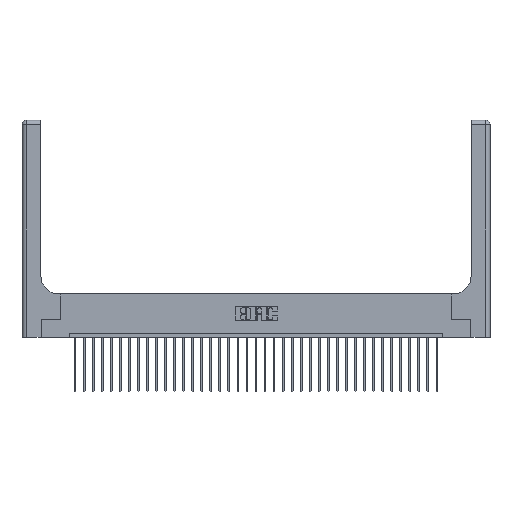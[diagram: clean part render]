
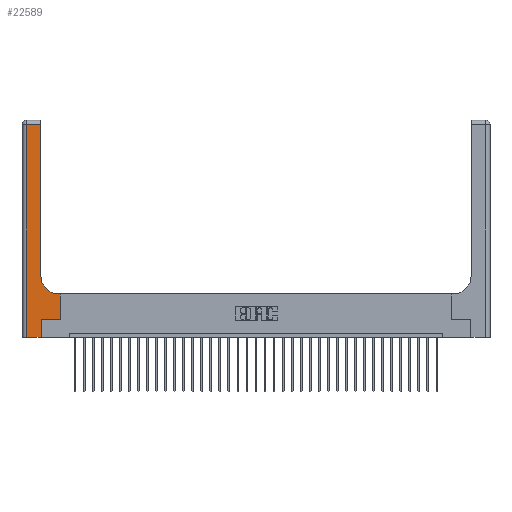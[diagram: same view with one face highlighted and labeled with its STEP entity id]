
A CAD part, top view. The second image highlights one B-rep face of the part: STEP entity #22589.
In plain terms, the highlighted planar face has unit normal (0, 0, 1).
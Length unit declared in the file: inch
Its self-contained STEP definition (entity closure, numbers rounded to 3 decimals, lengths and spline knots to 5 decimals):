
#271 = EDGE_CURVE ( 'NONE', #10063, #20399, #29861, .T. ) ;
#325 = DIRECTION ( 'NONE',  ( 0., 0., -1. ) ) ;
#635 = CARTESIAN_POINT ( 'NONE',  ( 0.06, 2.94, 0.37 ) ) ;
#3884 = EDGE_CURVE ( 'NONE', #7198, #19068, #24522, .T. ) ;
#4706 = VERTEX_POINT ( 'NONE', #23035 ) ;
#4895 = DIRECTION ( 'NONE',  ( -1., 0., 0. ) ) ;
#5053 = VECTOR ( 'NONE', #22862, 39.37008 ) ;
#5226 = CARTESIAN_POINT ( 'NONE',  ( 0.26, 2.94, 0.37 ) ) ;
#5548 = ORIENTED_EDGE ( 'NONE', *, *, #19573, .T. ) ;
#5899 = LINE ( 'NONE', #7981, #23345 ) ;
#5954 = LINE ( 'NONE', #9879, #23741 ) ;
#6757 = VECTOR ( 'NONE', #23575, 39.37008 ) ;
#7185 = PLANE ( 'NONE',  #28968 ) ;
#7198 = VERTEX_POINT ( 'NONE', #10456 ) ;
#7258 = CARTESIAN_POINT ( 'NONE',  ( 0., 2.94, 0.37 ) ) ;
#7278 = ORIENTED_EDGE ( 'NONE', *, *, #19802, .T. ) ;
#7500 = ORIENTED_EDGE ( 'NONE', *, *, #27510, .T. ) ;
#7981 = CARTESIAN_POINT ( 'NONE',  ( 0.26, 3., 0.37 ) ) ;
#8164 = DIRECTION ( 'NONE',  ( 0., 1., 0. ) ) ;
#8450 = DIRECTION ( 'NONE',  ( 1., 0., 0. ) ) ;
#8610 = VERTEX_POINT ( 'NONE', #23771 ) ;
#8743 = CARTESIAN_POINT ( 'NONE',  ( 0., 0., 0.37 ) ) ;
#9048 = CARTESIAN_POINT ( 'NONE',  ( 0.26, 0.85, 0.37 ) ) ;
#9879 = CARTESIAN_POINT ( 'NONE',  ( 0.26, 0.6, 0.37 ) ) ;
#10063 = VERTEX_POINT ( 'NONE', #18207 ) ;
#10200 = LINE ( 'NONE', #12173, #28010 ) ;
#10275 = CARTESIAN_POINT ( 'NONE',  ( 0.265, 0., 0.37 ) ) ;
#10456 = CARTESIAN_POINT ( 'NONE',  ( 0.265, 0.25, 0.37 ) ) ;
#12022 = CARTESIAN_POINT ( 'NONE',  ( 0.528, 0.25, 0.37 ) ) ;
#12166 = EDGE_LOOP ( 'NONE', ( #25432, #7500, #29569, #5548, #7278, #21839, #30677, #12741, #23522 ) ) ;
#12173 = CARTESIAN_POINT ( 'NONE',  ( 0.06, 3., 0.37 ) ) ;
#12741 = ORIENTED_EDGE ( 'NONE', *, *, #16975, .T. ) ;
#13682 = DIRECTION ( 'NONE',  ( 0., 0., -1. ) ) ;
#14010 = LINE ( 'NONE', #8743, #5053 ) ;
#15401 = CARTESIAN_POINT ( 'NONE',  ( 0.265, 0., 0.37 ) ) ;
#15419 = CARTESIAN_POINT ( 'NONE',  ( 0.528, 0.25, 0.37 ) ) ;
#16135 = VERTEX_POINT ( 'NONE', #5226 ) ;
#16975 = EDGE_CURVE ( 'NONE', #4706, #10063, #5954, .T. ) ;
#17598 = EDGE_CURVE ( 'NONE', #20399, #16135, #5899, .T. ) ;
#17746 = EDGE_CURVE ( 'NONE', #19068, #4706, #30760, .T. ) ;
#18207 = CARTESIAN_POINT ( 'NONE',  ( 0.51, 0.6, 0.37 ) ) ;
#19068 = VERTEX_POINT ( 'NONE', #12022 ) ;
#19573 = EDGE_CURVE ( 'NONE', #8610, #22750, #14010, .T. ) ;
#19642 = DIRECTION ( 'NONE',  ( -1., 0., 0. ) ) ;
#19802 = EDGE_CURVE ( 'NONE', #22750, #7198, #26176, .T. ) ;
#19907 = VECTOR ( 'NONE', #8164, 39.37008 ) ;
#20399 = VERTEX_POINT ( 'NONE', #9048 ) ;
#20532 = EDGE_CURVE ( 'NONE', #26271, #8610, #10200, .T. ) ;
#20753 = VECTOR ( 'NONE', #25188, 39.37008 ) ;
#21287 = DIRECTION ( 'NONE',  ( -1., 0., 0. ) ) ;
#21786 = DIRECTION ( 'NONE',  ( 0., -1., 0. ) ) ;
#21839 = ORIENTED_EDGE ( 'NONE', *, *, #3884, .T. ) ;
#22589 = ADVANCED_FACE ( 'NONE', ( #29532 ), #7185, .F. ) ;
#22750 = VERTEX_POINT ( 'NONE', #15401 ) ;
#22862 = DIRECTION ( 'NONE',  ( 1., 0., 0. ) ) ;
#22871 = CARTESIAN_POINT ( 'NONE',  ( 0.51, 0.85, 0.37 ) ) ;
#23035 = CARTESIAN_POINT ( 'NONE',  ( 0.528, 0.6, 0.37 ) ) ;
#23345 = VECTOR ( 'NONE', #26850, 39.37008 ) ;
#23522 = ORIENTED_EDGE ( 'NONE', *, *, #271, .T. ) ;
#23575 = DIRECTION ( 'NONE',  ( 1., 0., 0. ) ) ;
#23741 = VECTOR ( 'NONE', #19642, 39.37008 ) ;
#23771 = CARTESIAN_POINT ( 'NONE',  ( 0.06, 0., 0.37 ) ) ;
#23787 = CARTESIAN_POINT ( 'NONE',  ( 0., 3., 0.37 ) ) ;
#24386 = VECTOR ( 'NONE', #21287, 39.37008 ) ;
#24522 = LINE ( 'NONE', #28549, #6757 ) ;
#25188 = DIRECTION ( 'NONE',  ( 0., 1., 0. ) ) ;
#25432 = ORIENTED_EDGE ( 'NONE', *, *, #17598, .T. ) ;
#26176 = LINE ( 'NONE', #10275, #19907 ) ;
#26271 = VERTEX_POINT ( 'NONE', #635 ) ;
#26850 = DIRECTION ( 'NONE',  ( 0., 1., 0. ) ) ;
#27510 = EDGE_CURVE ( 'NONE', #16135, #26271, #30753, .T. ) ;
#28010 = VECTOR ( 'NONE', #21786, 39.37008 ) ;
#28549 = CARTESIAN_POINT ( 'NONE',  ( 0.265, 0.25, 0.37 ) ) ;
#28968 = AXIS2_PLACEMENT_3D ( 'NONE', #23787, #325, #4895 ) ;
#29116 = AXIS2_PLACEMENT_3D ( 'NONE', #22871, #13682, #8450 ) ;
#29532 = FACE_OUTER_BOUND ( 'NONE', #12166, .T. ) ;
#29569 = ORIENTED_EDGE ( 'NONE', *, *, #20532, .T. ) ;
#29861 = CIRCLE ( 'NONE', #29116, 0.25 ) ;
#30677 = ORIENTED_EDGE ( 'NONE', *, *, #17746, .T. ) ;
#30753 = LINE ( 'NONE', #7258, #24386 ) ;
#30760 = LINE ( 'NONE', #15419, #20753 ) ;
